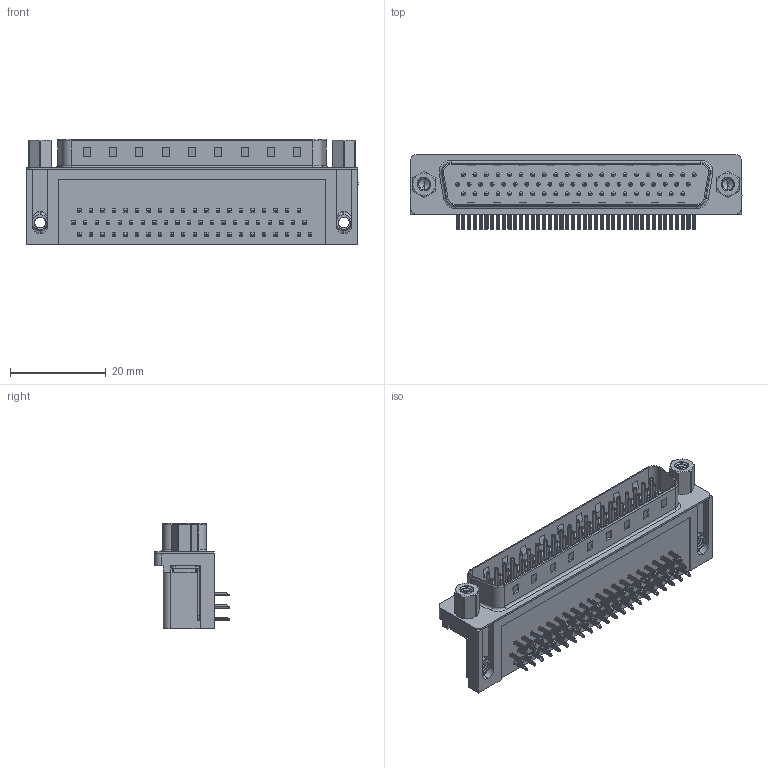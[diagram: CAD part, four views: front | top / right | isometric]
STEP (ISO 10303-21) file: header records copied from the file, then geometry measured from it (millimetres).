
FILE_DESCRIPTION (( 'STEP AP203' ), '1' );
FILE_NAME ('633-062-363-053.STEP', '2018-11-09T03:59:50', ( '' ), ( '' ), 'SwSTEP 2.0', 'SolidWorks 2016', '' );
FILE_SCHEMA (( 'CONFIG_CONTROL_DESIGN' ));
Length unit declared in the file: millimetre
Products named in the file (9): 633 Contact Top; 633 4-40 Threaded Board Mount; 633 4-40 Threaded Rivet; 633 4-40 Hex Standoff; 633-062-363-053; 633 Housing_62 Contact; 633 Shell_62 Contact; 633 Contact Bottom; 633 Contact Middle
Assembly tree (70 placements, depth 2):
  633-062-363-053
    633 Housing_62 Contact
    633 Shell_62 Contact
    633 Contact Bottom  x20
    633 Contact Middle  x21
    633 Contact Top  x21
    633 4-40 Threaded Board Mount  x2
    633 4-40 Threaded Rivet  x2
    633 4-40 Hex Standoff  x2
Bounding box: 69.4 x 15.73 x 22.1 mm (x, y, z)
Volume: 11268.6 mm3; surface area: 13938.2 mm2
Topology: 70 solids, 70 shells, 5226 faces, 12894 edges, 7941 vertices
Faces by surface type: plane 3235, cylinder 1518, torus 415, cone 34, bspline 24
Entity records: 41330 total; most frequent: CARTESIAN_POINT 11486, DIRECTION 5689, ORIENTED_EDGE 5542, EDGE_CURVE 2771, VECTOR 1921, LINE 1921, AXIS2_PLACEMENT_3D 1884, VERTEX_POINT 1791
